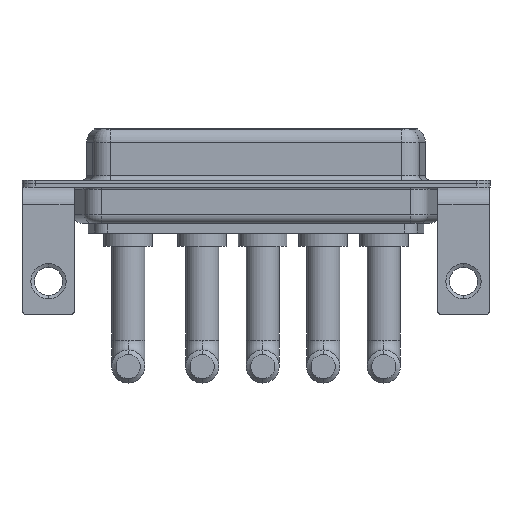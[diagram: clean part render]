
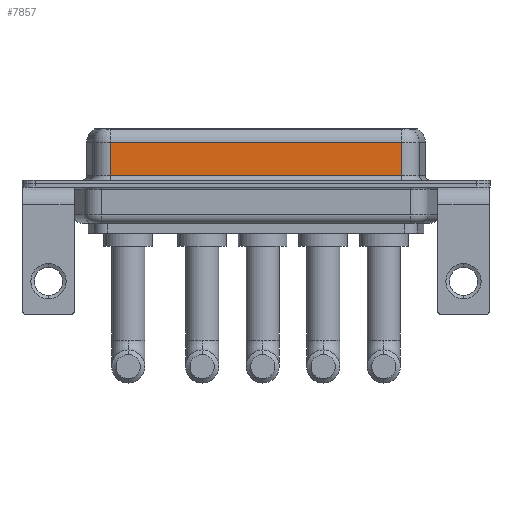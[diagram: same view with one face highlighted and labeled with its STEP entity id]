
A CAD part, front view. The second image highlights one B-rep face of the part: STEP entity #7857.
In plain terms, the highlighted planar face has unit normal (0, -1, 0).
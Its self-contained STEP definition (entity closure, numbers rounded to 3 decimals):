
#668 = ORIENTED_EDGE ( 'NONE', *, *, #1790, .T. ) ;
#867 = ORIENTED_EDGE ( 'NONE', *, *, #13112, .T. ) ;
#1790 = EDGE_CURVE ( 'NONE', #9914, #11896, #6914, .T. ) ;
#2369 = ORIENTED_EDGE ( 'NONE', *, *, #13107, .T. ) ;
#2422 = LINE ( 'NONE', #11836, #7390 ) ;
#2671 = DIRECTION ( 'NONE',  ( 0., 0., -1. ) ) ;
#2758 = CARTESIAN_POINT ( 'NONE',  ( 7.013, -3.95, 6.4 ) ) ;
#2845 = ORIENTED_EDGE ( 'NONE', *, *, #6509, .F. ) ;
#3257 = VECTOR ( 'NONE', #6578, 1000. ) ;
#3702 = FACE_OUTER_BOUND ( 'NONE', #7978, .T. ) ;
#4005 = VERTEX_POINT ( 'NONE', #11397 ) ;
#4631 = VECTOR ( 'NONE', #2671, 1000. ) ;
#5563 = LINE ( 'NONE', #8423, #3257 ) ;
#6002 = CARTESIAN_POINT ( 'NONE',  ( 40.037, -3.95, 6.4 ) ) ;
#6509 = EDGE_CURVE ( 'NONE', #7152, #4005, #9823, .T. ) ;
#6578 = DIRECTION ( 'NONE',  ( -1., 0., 0. ) ) ;
#6914 = LINE ( 'NONE', #2758, #12605 ) ;
#6960 = CARTESIAN_POINT ( 'NONE',  ( 40.037, -3.95, 6.4 ) ) ;
#7152 = VERTEX_POINT ( 'NONE', #7662 ) ;
#7390 = VECTOR ( 'NONE', #11557, 1000. ) ;
#7662 = CARTESIAN_POINT ( 'NONE',  ( 40.037, -3.95, 4.65 ) ) ;
#7857 = ADVANCED_FACE ( 'NONE', ( #3702 ), #8054, .F. ) ;
#7978 = EDGE_LOOP ( 'NONE', ( #2845, #867, #668, #2369 ) ) ;
#8054 = PLANE ( 'NONE',  #9412 ) ;
#8423 = CARTESIAN_POINT ( 'NONE',  ( 40.037, -3.95, 4.65 ) ) ;
#9412 = AXIS2_PLACEMENT_3D ( 'NONE', #6002, #12010, #10028 ) ;
#9823 = LINE ( 'NONE', #6960, #4631 ) ;
#9914 = VERTEX_POINT ( 'NONE', #13201 ) ;
#10028 = DIRECTION ( 'NONE',  ( 0., 0., 1. ) ) ;
#11009 = DIRECTION ( 'NONE',  ( 0., 0., -1. ) ) ;
#11397 = CARTESIAN_POINT ( 'NONE',  ( 40.037, -3.95, 0.9 ) ) ;
#11557 = DIRECTION ( 'NONE',  ( 1., 0., 0. ) ) ;
#11836 = CARTESIAN_POINT ( 'NONE',  ( 40.037, -3.95, 0.9 ) ) ;
#11896 = VERTEX_POINT ( 'NONE', #12443 ) ;
#12010 = DIRECTION ( 'NONE',  ( 0., 1., 0. ) ) ;
#12443 = CARTESIAN_POINT ( 'NONE',  ( 7.013, -3.95, 0.9 ) ) ;
#12605 = VECTOR ( 'NONE', #11009, 1000. ) ;
#13107 = EDGE_CURVE ( 'NONE', #11896, #4005, #2422, .T. ) ;
#13112 = EDGE_CURVE ( 'NONE', #7152, #9914, #5563, .T. ) ;
#13201 = CARTESIAN_POINT ( 'NONE',  ( 7.013, -3.95, 4.65 ) ) ;
